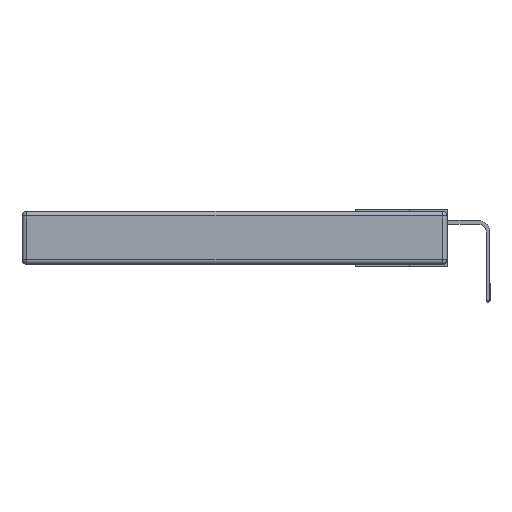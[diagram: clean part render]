
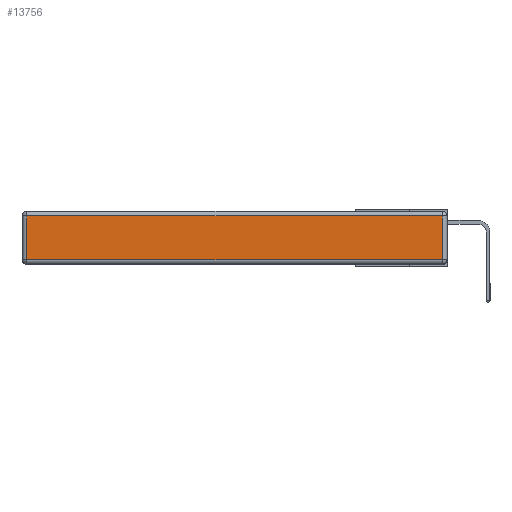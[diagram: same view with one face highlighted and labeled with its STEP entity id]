
A CAD part, left-side view. The second image highlights one B-rep face of the part: STEP entity #13756.
In plain terms, the highlighted planar face has unit normal (-1, 0, 0).
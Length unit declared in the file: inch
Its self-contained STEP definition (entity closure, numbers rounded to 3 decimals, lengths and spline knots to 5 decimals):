
#628 = LINE ( 'NONE', #23807, #9707 ) ;
#928 = CARTESIAN_POINT ( 'NONE',  ( 0., 0.03, -0.03 ) ) ;
#1783 = CARTESIAN_POINT ( 'NONE',  ( 0., 0., -0.343 ) ) ;
#2343 = VECTOR ( 'NONE', #4132, 39.37008 ) ;
#2578 = ORIENTED_EDGE ( 'NONE', *, *, #8185, .T. ) ;
#2936 = VECTOR ( 'NONE', #18021, 39.37008 ) ;
#3575 = VECTOR ( 'NONE', #15018, 39.37008 ) ;
#4132 = DIRECTION ( 'NONE',  ( 0., 1., 0. ) ) ;
#4297 = DIRECTION ( 'NONE',  ( 0., 0., -1. ) ) ;
#5187 = CARTESIAN_POINT ( 'NONE',  ( 0., 0., -0.313 ) ) ;
#5939 = EDGE_LOOP ( 'NONE', ( #9427, #12145, #2578, #9206 ) ) ;
#8185 = EDGE_CURVE ( 'NONE', #10278, #9839, #21877, .T. ) ;
#8876 = FACE_OUTER_BOUND ( 'NONE', #5939, .T. ) ;
#9206 = ORIENTED_EDGE ( 'NONE', *, *, #14985, .T. ) ;
#9427 = ORIENTED_EDGE ( 'NONE', *, *, #12568, .T. ) ;
#9707 = VECTOR ( 'NONE', #4297, 39.37008 ) ;
#9839 = VERTEX_POINT ( 'NONE', #24290 ) ;
#10278 = VERTEX_POINT ( 'NONE', #928 ) ;
#10322 = CARTESIAN_POINT ( 'NONE',  ( 0., 0.03, -0.343 ) ) ;
#11303 = LINE ( 'NONE', #5187, #2936 ) ;
#12145 = ORIENTED_EDGE ( 'NONE', *, *, #16686, .T. ) ;
#12412 = PLANE ( 'NONE',  #25584 ) ;
#12568 = EDGE_CURVE ( 'NONE', #18814, #15088, #11303, .T. ) ;
#12577 = CARTESIAN_POINT ( 'NONE',  ( 0., 2.72, -0.313 ) ) ;
#13756 = ADVANCED_FACE ( 'NONE', ( #8876 ), #12412, .T. ) ;
#14373 = LINE ( 'NONE', #10322, #3575 ) ;
#14985 = EDGE_CURVE ( 'NONE', #9839, #18814, #628, .T. ) ;
#15018 = DIRECTION ( 'NONE',  ( 0., 0., 1. ) ) ;
#15088 = VERTEX_POINT ( 'NONE', #26057 ) ;
#16686 = EDGE_CURVE ( 'NONE', #15088, #10278, #14373, .T. ) ;
#16849 = DIRECTION ( 'NONE',  ( 0., 0., 1. ) ) ;
#18021 = DIRECTION ( 'NONE',  ( 0., -1., 0. ) ) ;
#18814 = VERTEX_POINT ( 'NONE', #12577 ) ;
#21877 = LINE ( 'NONE', #23441, #2343 ) ;
#23441 = CARTESIAN_POINT ( 'NONE',  ( 0., 2.75, -0.03 ) ) ;
#23807 = CARTESIAN_POINT ( 'NONE',  ( 0., 2.72, -0.343 ) ) ;
#24290 = CARTESIAN_POINT ( 'NONE',  ( 0., 2.72, -0.03 ) ) ;
#25584 = AXIS2_PLACEMENT_3D ( 'NONE', #1783, #27484, #16849 ) ;
#26057 = CARTESIAN_POINT ( 'NONE',  ( 0., 0.03, -0.313 ) ) ;
#27484 = DIRECTION ( 'NONE',  ( -1., 0., 0. ) ) ;
